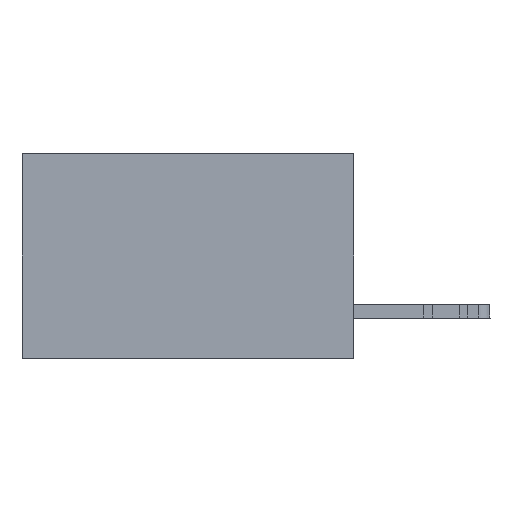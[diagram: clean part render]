
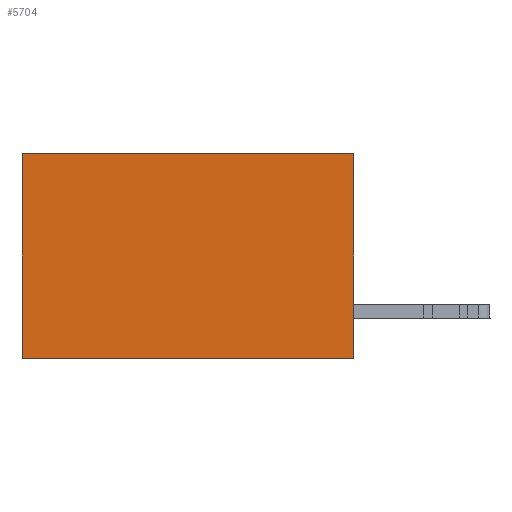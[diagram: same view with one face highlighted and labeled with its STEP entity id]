
A CAD part, left-side view. The second image highlights one B-rep face of the part: STEP entity #5704.
In plain terms, the highlighted planar face has unit normal (-1, 0, 0).
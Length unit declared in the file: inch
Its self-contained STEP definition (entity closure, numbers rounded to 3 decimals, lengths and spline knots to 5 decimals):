
#1187 = LINE ( 'NONE', #34099, #37509 ) ;
#3420 = DIRECTION ( 'NONE',  ( 0., 0., -1. ) ) ;
#5704 = ADVANCED_FACE ( 'NONE', ( #44505 ), #15465, .F. ) ;
#5765 = ORIENTED_EDGE ( 'NONE', *, *, #10600, .F. ) ;
#6252 = LINE ( 'NONE', #30119, #21643 ) ;
#8100 = EDGE_CURVE ( 'NONE', #35000, #20433, #17536, .T. ) ;
#8143 = VECTOR ( 'NONE', #32988, 39.37008 ) ;
#9072 = DIRECTION ( 'NONE',  ( 0., 1., 0. ) ) ;
#10304 = AXIS2_PLACEMENT_3D ( 'NONE', #40087, #19029, #43554 ) ;
#10600 = EDGE_CURVE ( 'NONE', #33320, #41386, #6252, .T. ) ;
#11825 = CARTESIAN_POINT ( 'NONE',  ( 0.2875, 0., 0. ) ) ;
#12280 = CARTESIAN_POINT ( 'NONE',  ( 0.2875, 0., -0.37 ) ) ;
#12889 = EDGE_CURVE ( 'NONE', #20433, #41386, #1187, .T. ) ;
#14873 = CARTESIAN_POINT ( 'NONE',  ( 0.2875, 0.6, 0. ) ) ;
#15191 = ORIENTED_EDGE ( 'NONE', *, *, #8100, .T. ) ;
#15465 = PLANE ( 'NONE',  #10304 ) ;
#17536 = LINE ( 'NONE', #21951, #8143 ) ;
#19029 = DIRECTION ( 'NONE',  ( 1., 0., 0. ) ) ;
#20433 = VERTEX_POINT ( 'NONE', #14873 ) ;
#20680 = CARTESIAN_POINT ( 'NONE',  ( 0.2875, 0.6, -0.37 ) ) ;
#20830 = LINE ( 'NONE', #11825, #23060 ) ;
#21643 = VECTOR ( 'NONE', #9072, 39.37008 ) ;
#21951 = CARTESIAN_POINT ( 'NONE',  ( 0.2875, 0., 0. ) ) ;
#23060 = VECTOR ( 'NONE', #3420, 39.37008 ) ;
#24447 = CARTESIAN_POINT ( 'NONE',  ( 0.2875, 0., 0. ) ) ;
#28121 = EDGE_LOOP ( 'NONE', ( #42695, #5765, #30498, #15191 ) ) ;
#29425 = EDGE_CURVE ( 'NONE', #35000, #33320, #20830, .T. ) ;
#30119 = CARTESIAN_POINT ( 'NONE',  ( 0.2875, 0., -0.37 ) ) ;
#30498 = ORIENTED_EDGE ( 'NONE', *, *, #29425, .F. ) ;
#32988 = DIRECTION ( 'NONE',  ( 0., 1., 0. ) ) ;
#33320 = VERTEX_POINT ( 'NONE', #12280 ) ;
#34099 = CARTESIAN_POINT ( 'NONE',  ( 0.2875, 0.6, 0. ) ) ;
#35000 = VERTEX_POINT ( 'NONE', #24447 ) ;
#37509 = VECTOR ( 'NONE', #41157, 39.37008 ) ;
#40087 = CARTESIAN_POINT ( 'NONE',  ( 0.2875, 0., 0. ) ) ;
#41157 = DIRECTION ( 'NONE',  ( 0., 0., -1. ) ) ;
#41386 = VERTEX_POINT ( 'NONE', #20680 ) ;
#42695 = ORIENTED_EDGE ( 'NONE', *, *, #12889, .T. ) ;
#43554 = DIRECTION ( 'NONE',  ( 0., 0., -1. ) ) ;
#44505 = FACE_OUTER_BOUND ( 'NONE', #28121, .T. ) ;
